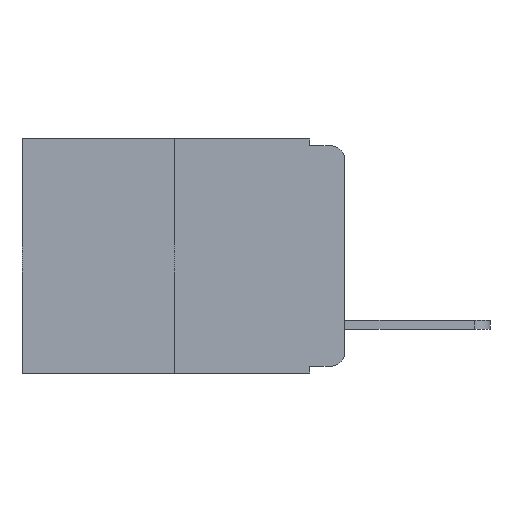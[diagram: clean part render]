
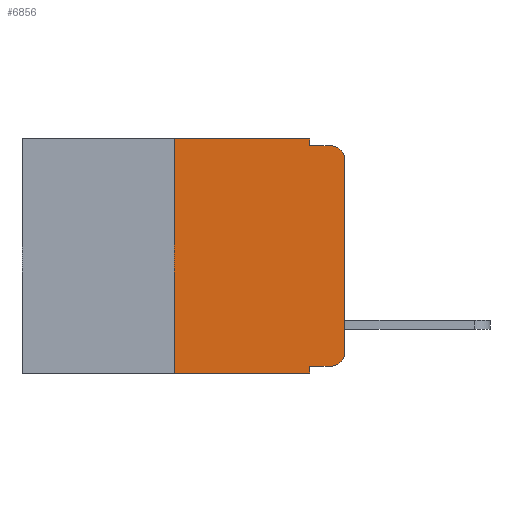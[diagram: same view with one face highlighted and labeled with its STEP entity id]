
A CAD part, left-side view. The second image highlights one B-rep face of the part: STEP entity #6856.
In plain terms, the highlighted planar face has unit normal (-1, 0, 0).
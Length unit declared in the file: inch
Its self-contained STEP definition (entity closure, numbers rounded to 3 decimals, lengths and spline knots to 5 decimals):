
#536 = DIRECTION ( 'NONE',  ( 0., 0., -1. ) ) ;
#771 = VECTOR ( 'NONE', #4854, 39.37008 ) ;
#936 = VERTEX_POINT ( 'NONE', #1444 ) ;
#1000 = DIRECTION ( 'NONE',  ( 0., -1., 0. ) ) ;
#1034 = AXIS2_PLACEMENT_3D ( 'NONE', #5399, #14362, #4183 ) ;
#1261 = CARTESIAN_POINT ( 'NONE',  ( 0., 0.25, 0. ) ) ;
#1334 = VECTOR ( 'NONE', #1000, 39.37008 ) ;
#1444 = CARTESIAN_POINT ( 'NONE',  ( 0., 0.25, -0.343 ) ) ;
#1450 = VECTOR ( 'NONE', #14408, 39.37008 ) ;
#1464 = ORIENTED_EDGE ( 'NONE', *, *, #13573, .F. ) ;
#1626 = EDGE_CURVE ( 'NONE', #3211, #5815, #9353, .T. ) ;
#1886 = VERTEX_POINT ( 'NONE', #14314 ) ;
#2029 = CARTESIAN_POINT ( 'NONE',  ( 0., 0.473, 0. ) ) ;
#2110 = EDGE_CURVE ( 'NONE', #5132, #2435, #8616, .T. ) ;
#2162 = CARTESIAN_POINT ( 'NONE',  ( 0., 0.051, -0.343 ) ) ;
#2308 = LINE ( 'NONE', #9858, #10418 ) ;
#2435 = VERTEX_POINT ( 'NONE', #2162 ) ;
#2479 = CARTESIAN_POINT ( 'NONE',  ( 0., 0.02, -0.313 ) ) ;
#2485 = VECTOR ( 'NONE', #2976, 39.37008 ) ;
#2938 = ORIENTED_EDGE ( 'NONE', *, *, #7521, .F. ) ;
#2976 = DIRECTION ( 'NONE',  ( 0., -1., 0. ) ) ;
#3180 = EDGE_CURVE ( 'NONE', #9299, #14217, #12811, .T. ) ;
#3211 = VERTEX_POINT ( 'NONE', #10511 ) ;
#3236 = VECTOR ( 'NONE', #14219, 39.37008 ) ;
#3686 = VERTEX_POINT ( 'NONE', #1261 ) ;
#3843 = CARTESIAN_POINT ( 'NONE',  ( 0., 0., 0. ) ) ;
#3938 = EDGE_LOOP ( 'NONE', ( #14142, #10539, #6639, #2938, #4878, #1464, #11345, #8464, #11334, #9849 ) ) ;
#4136 = PLANE ( 'NONE',  #11170 ) ;
#4183 = DIRECTION ( 'NONE',  ( 0., 0., -1. ) ) ;
#4463 = VERTEX_POINT ( 'NONE', #11513 ) ;
#4854 = DIRECTION ( 'NONE',  ( 0., -1., 0. ) ) ;
#4878 = ORIENTED_EDGE ( 'NONE', *, *, #10369, .F. ) ;
#4953 = DIRECTION ( 'NONE',  ( 0., 0., -1. ) ) ;
#5132 = VERTEX_POINT ( 'NONE', #6554 ) ;
#5399 = CARTESIAN_POINT ( 'NONE',  ( 0., 0.02, -0.03 ) ) ;
#5486 = DIRECTION ( 'NONE',  ( 0., 0., -1. ) ) ;
#5773 = DIRECTION ( 'NONE',  ( 1., 0., 0. ) ) ;
#5815 = VERTEX_POINT ( 'NONE', #8797 ) ;
#5875 = LINE ( 'NONE', #6983, #2485 ) ;
#6554 = CARTESIAN_POINT ( 'NONE',  ( 0., 0.051, -0.333 ) ) ;
#6639 = ORIENTED_EDGE ( 'NONE', *, *, #1626, .F. ) ;
#6691 = VECTOR ( 'NONE', #11840, 39.37008 ) ;
#6856 = ADVANCED_FACE ( 'NONE', ( #12515 ), #4136, .F. ) ;
#6983 = CARTESIAN_POINT ( 'NONE',  ( 0., 0.473, -0.343 ) ) ;
#7521 = EDGE_CURVE ( 'NONE', #4463, #3211, #2308, .T. ) ;
#7620 = EDGE_CURVE ( 'NONE', #936, #2435, #5875, .T. ) ;
#7813 = LINE ( 'NONE', #11611, #1334 ) ;
#8281 = LINE ( 'NONE', #13320, #1450 ) ;
#8464 = ORIENTED_EDGE ( 'NONE', *, *, #2110, .F. ) ;
#8616 = LINE ( 'NONE', #9658, #14213 ) ;
#8797 = CARTESIAN_POINT ( 'NONE',  ( 0., 0.02, -0.01 ) ) ;
#8962 = EDGE_CURVE ( 'NONE', #1886, #5815, #11095, .T. ) ;
#9299 = VERTEX_POINT ( 'NONE', #9900 ) ;
#9353 = LINE ( 'NONE', #13978, #3236 ) ;
#9416 = LINE ( 'NONE', #3843, #6691 ) ;
#9658 = CARTESIAN_POINT ( 'NONE',  ( 0., 0.051, 0. ) ) ;
#9849 = ORIENTED_EDGE ( 'NONE', *, *, #3180, .T. ) ;
#9858 = CARTESIAN_POINT ( 'NONE',  ( 0., 0.051, 0. ) ) ;
#9900 = CARTESIAN_POINT ( 'NONE',  ( 0., 0.02, -0.333 ) ) ;
#9977 = LINE ( 'NONE', #10603, #771 ) ;
#10112 = EDGE_CURVE ( 'NONE', #5132, #9299, #7813, .T. ) ;
#10369 = EDGE_CURVE ( 'NONE', #3686, #4463, #9977, .T. ) ;
#10418 = VECTOR ( 'NONE', #4953, 39.37008 ) ;
#10437 = DIRECTION ( 'NONE',  ( 0., 0., -1. ) ) ;
#10511 = CARTESIAN_POINT ( 'NONE',  ( 0., 0.051, -0.01 ) ) ;
#10539 = ORIENTED_EDGE ( 'NONE', *, *, #8962, .T. ) ;
#10603 = CARTESIAN_POINT ( 'NONE',  ( 0., 0.473, 0. ) ) ;
#11069 = EDGE_CURVE ( 'NONE', #14217, #1886, #9416, .T. ) ;
#11095 = CIRCLE ( 'NONE', #1034, 0.02 ) ;
#11170 = AXIS2_PLACEMENT_3D ( 'NONE', #2029, #5773, #5486 ) ;
#11334 = ORIENTED_EDGE ( 'NONE', *, *, #10112, .T. ) ;
#11345 = ORIENTED_EDGE ( 'NONE', *, *, #7620, .T. ) ;
#11513 = CARTESIAN_POINT ( 'NONE',  ( 0., 0.051, 0. ) ) ;
#11611 = CARTESIAN_POINT ( 'NONE',  ( 0., 0.051, -0.333 ) ) ;
#11840 = DIRECTION ( 'NONE',  ( 0., 0., 1. ) ) ;
#12074 = DIRECTION ( 'NONE',  ( -1., 0., 0. ) ) ;
#12515 = FACE_OUTER_BOUND ( 'NONE', #3938, .T. ) ;
#12520 = AXIS2_PLACEMENT_3D ( 'NONE', #2479, #12074, #536 ) ;
#12811 = CIRCLE ( 'NONE', #12520, 0.02 ) ;
#13320 = CARTESIAN_POINT ( 'NONE',  ( 0., 0.25, 0. ) ) ;
#13573 = EDGE_CURVE ( 'NONE', #936, #3686, #8281, .T. ) ;
#13978 = CARTESIAN_POINT ( 'NONE',  ( 0., 0.051, -0.01 ) ) ;
#14142 = ORIENTED_EDGE ( 'NONE', *, *, #11069, .T. ) ;
#14213 = VECTOR ( 'NONE', #10437, 39.37008 ) ;
#14217 = VERTEX_POINT ( 'NONE', #14565 ) ;
#14219 = DIRECTION ( 'NONE',  ( 0., -1., 0. ) ) ;
#14314 = CARTESIAN_POINT ( 'NONE',  ( 0., 0., -0.03 ) ) ;
#14362 = DIRECTION ( 'NONE',  ( -1., 0., 0. ) ) ;
#14408 = DIRECTION ( 'NONE',  ( 0., 0., 1. ) ) ;
#14565 = CARTESIAN_POINT ( 'NONE',  ( 0., 0., -0.313 ) ) ;
